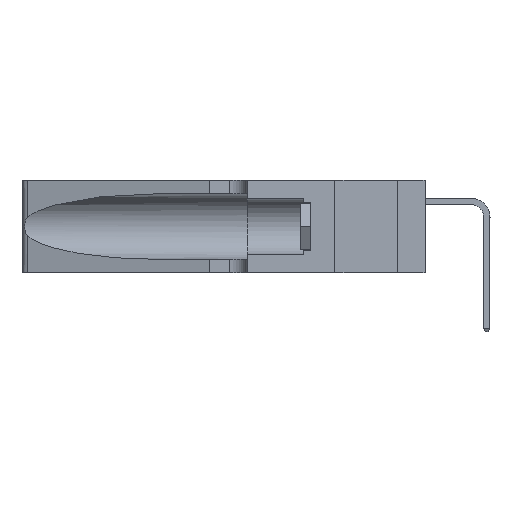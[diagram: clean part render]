
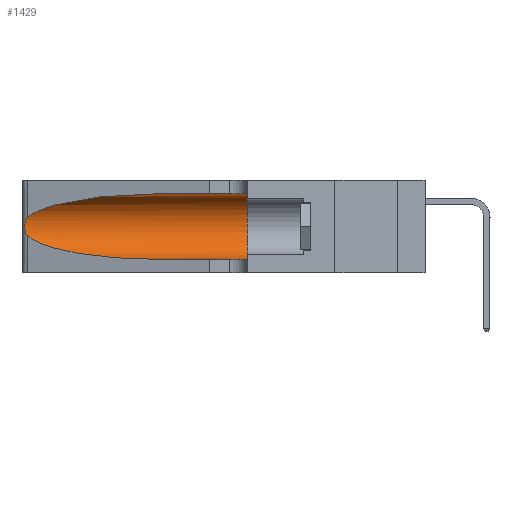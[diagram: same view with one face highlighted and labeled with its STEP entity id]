
A CAD part, left-side view. The second image highlights one B-rep face of the part: STEP entity #1429.
In plain terms, the highlighted cylindrical face has radius 3.308 mm (diameter 6.617 mm), a partial arc.
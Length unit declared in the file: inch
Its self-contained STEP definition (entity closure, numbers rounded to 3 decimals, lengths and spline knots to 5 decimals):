
#145 = EDGE_CURVE ( 'NONE', #21900, #17245, #22277, .T. ) ;
#1429 = ADVANCED_FACE ( 'NONE', ( #3001 ), #17709, .F. ) ;
#2078 = CARTESIAN_POINT ( 'NONE',  ( 0.1305, 0.72297, 0.31525 ) ) ;
#2117 = EDGE_CURVE ( 'NONE', #7076, #19915, #17350, .T. ) ;
#2166 = CARTESIAN_POINT ( 'NONE',  ( 0.1305, 0.72297, 0.05475 ) ) ;
#2461 = VERTEX_POINT ( 'NONE', #2166 ) ;
#3001 = FACE_OUTER_BOUND ( 'NONE', #10899, .T. ) ;
#3162 = ORIENTED_EDGE ( 'NONE', *, *, #2117, .F. ) ;
#3511 = CARTESIAN_POINT ( 'NONE',  ( 0.1305, 0.72297, 0.31525 ) ) ;
#3664 = CARTESIAN_POINT ( 'NONE',  ( 0.25555, 1.22993, 0.14849 ) ) ;
#4145 = ORIENTED_EDGE ( 'NONE', *, *, #145, .T. ) ;
#4586 = CARTESIAN_POINT ( 'NONE',  ( 0.1305, 1.61858, 0.185 ) ) ;
#4876 = EDGE_CURVE ( 'NONE', #19915, #9375, #7615, .T. ) ;
#4980 = CARTESIAN_POINT ( 'NONE',  ( 0.1305, 1.61858, 0.31525 ) ) ;
#5065 = CARTESIAN_POINT ( 'NONE',  ( 0.1305, 0.35, 0.185 ) ) ;
#6415 = CARTESIAN_POINT ( 'NONE',  ( 0.26017, 1.23833, 0.17102 ) ) ;
#6490 = EDGE_CURVE ( 'NONE', #2461, #9375, #25960, .T. ) ;
#6996 = DIRECTION ( 'NONE',  ( 0., -1., 0. ) ) ;
#7068 = DIRECTION ( 'NONE',  ( 0., 0., 1. ) ) ;
#7076 = VERTEX_POINT ( 'NONE', #2078 ) ;
#7597 = CARTESIAN_POINT ( 'NONE',  ( 0.1305, 0.35, 0.05475 ) ) ;
#7615 = CIRCLE ( 'NONE', #20147, 0.13025 ) ;
#8612 = DIRECTION ( 'NONE',  ( 0., -1., 0. ) ) ;
#9375 = VERTEX_POINT ( 'NONE', #7597 ) ;
#9551 = CARTESIAN_POINT ( 'NONE',  ( 0.25487, 1.22718, 0.22369 ) ) ;
#9977 = CARTESIAN_POINT ( 'NONE',  ( 0.18966, 0.96281, 0.05475 ) ) ;
#10034 = VECTOR ( 'NONE', #16381, 39.37008 ) ;
#10650 = CARTESIAN_POINT ( 'NONE',  ( 0.25856, 1.23593, 0.16098 ) ) ;
#10899 = EDGE_LOOP ( 'NONE', ( #11938, #4145, #19584, #22530, #22854, #3162 ) ) ;
#10953 = CARTESIAN_POINT ( 'NONE',  ( 0.1305, 0.35, 0.31525 ) ) ;
#11434 = VECTOR ( 'NONE', #6996, 39.37008 ) ;
#11582 = CARTESIAN_POINT ( 'NONE',  ( 0.25487, 1.22718, 0.22369 ) ) ;
#11670 = CARTESIAN_POINT ( 'NONE',  ( 0.25639, 1.23184, 0.21858 ) ) ;
#11758 = AXIS2_PLACEMENT_3D ( 'NONE', #4586, #8612, #18566 ) ;
#11938 = ORIENTED_EDGE ( 'NONE', *, *, #24381, .T. ) ;
#12125 = CARTESIAN_POINT ( 'NONE',  ( 0.25639, 1.23186, 0.15144 ) ) ;
#12550 = CARTESIAN_POINT ( 'NONE',  ( 0.25789, 1.23486, 0.15765 ) ) ;
#14373 = CARTESIAN_POINT ( 'NONE',  ( 0.1305, 1.61858, 0.05475 ) ) ;
#15007 = CARTESIAN_POINT ( 'NONE',  ( 0.26075, 1.23896, 0.19203 ) ) ;
#15475 = CARTESIAN_POINT ( 'NONE',  ( 0.18966, 0.96281, 0.31525 ) ) ;
#15700 =( BOUNDED_CURVE ( )  B_SPLINE_CURVE ( 3, ( #19907, #21947, #9977, #23949 ),
 .UNSPECIFIED., .F., .F. ) 
 B_SPLINE_CURVE_WITH_KNOTS ( ( 4, 4 ),
 ( 3.44316, 4.71239 ),
 .UNSPECIFIED. ) 
 CURVE ( )  GEOMETRIC_REPRESENTATION_ITEM ( )  RATIONAL_B_SPLINE_CURVE ( ( 1., 0.87, 0.87, 1. ) ) 
 REPRESENTATION_ITEM ( '' )  );
#16231 = EDGE_CURVE ( 'NONE', #17245, #2461, #15700, .T. ) ;
#16381 = DIRECTION ( 'NONE',  ( 0., -1., 0. ) ) ;
#17245 = VERTEX_POINT ( 'NONE', #20999 ) ;
#17350 = LINE ( 'NONE', #4980, #11434 ) ;
#17547 = CARTESIAN_POINT ( 'NONE',  ( 0.25854, 1.2359, 0.20912 ) ) ;
#17605 = CARTESIAN_POINT ( 'NONE',  ( 0.25787, 1.23484, 0.2124 ) ) ;
#17709 = CYLINDRICAL_SURFACE ( 'NONE', #11758, 0.13025 ) ;
#18566 = DIRECTION ( 'NONE',  ( 0., 0., -1. ) ) ;
#19052 = DIRECTION ( 'NONE',  ( 0., 1., 0. ) ) ;
#19584 = ORIENTED_EDGE ( 'NONE', *, *, #16231, .T. ) ;
#19907 = CARTESIAN_POINT ( 'NONE',  ( 0.25487, 1.22718, 0.14631 ) ) ;
#19915 = VERTEX_POINT ( 'NONE', #10953 ) ;
#20147 = AXIS2_PLACEMENT_3D ( 'NONE', #5065, #19052, #7068 ) ;
#20830 = CARTESIAN_POINT ( 'NONE',  ( 0.25555, 1.22994, 0.2215 ) ) ;
#20999 = CARTESIAN_POINT ( 'NONE',  ( 0.25487, 1.22718, 0.14631 ) ) ;
#21515 = CARTESIAN_POINT ( 'NONE',  ( 0.2373, 1.15595, 0.28018 ) ) ;
#21631 = CARTESIAN_POINT ( 'NONE',  ( 0.25487, 1.22718, 0.22369 ) ) ;
#21900 = VERTEX_POINT ( 'NONE', #21631 ) ;
#21947 = CARTESIAN_POINT ( 'NONE',  ( 0.2373, 1.15595, 0.08982 ) ) ;
#22277 = B_SPLINE_CURVE_WITH_KNOTS ( 'NONE', 3,
 ( #11582, #20830, #11670, #17605, #17547, #22956, #15007, #25850, #6415, #10650, #12550, #12125, #3664, #23498 ),
 .UNSPECIFIED., .F., .F.,
 ( 4, 2, 2, 2, 2, 2, 4 ),
 ( 0., 0.00027, 0.00053, 0.00107, 0.0016, 0.00187, 0.00214 ),
 .UNSPECIFIED. ) ;
#22530 = ORIENTED_EDGE ( 'NONE', *, *, #6490, .T. ) ;
#22854 = ORIENTED_EDGE ( 'NONE', *, *, #4876, .F. ) ;
#22956 = CARTESIAN_POINT ( 'NONE',  ( 0.26018, 1.23835, 0.19895 ) ) ;
#23080 =( BOUNDED_CURVE ( )  B_SPLINE_CURVE ( 3, ( #3511, #15475, #21515, #9551 ),
 .UNSPECIFIED., .F., .F. ) 
 B_SPLINE_CURVE_WITH_KNOTS ( ( 4, 4 ),
 ( 1.5708, 2.84003 ),
 .UNSPECIFIED. ) 
 CURVE ( )  GEOMETRIC_REPRESENTATION_ITEM ( )  RATIONAL_B_SPLINE_CURVE ( ( 1., 0.87, 0.87, 1. ) ) 
 REPRESENTATION_ITEM ( '' )  );
#23498 = CARTESIAN_POINT ( 'NONE',  ( 0.25487, 1.22718, 0.14631 ) ) ;
#23949 = CARTESIAN_POINT ( 'NONE',  ( 0.1305, 0.72297, 0.05475 ) ) ;
#24381 = EDGE_CURVE ( 'NONE', #7076, #21900, #23080, .T. ) ;
#25850 = CARTESIAN_POINT ( 'NONE',  ( 0.26075, 1.23896, 0.178 ) ) ;
#25960 = LINE ( 'NONE', #14373, #10034 ) ;
